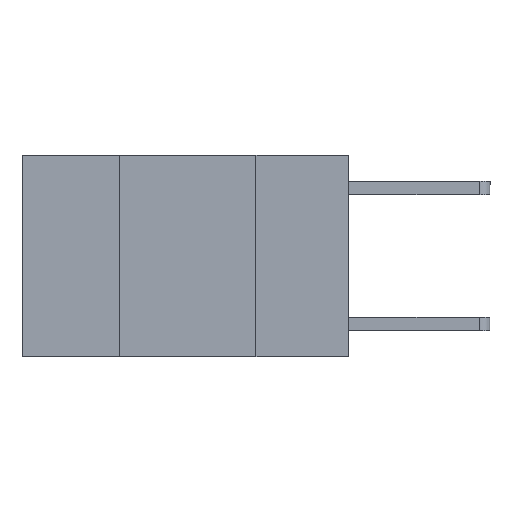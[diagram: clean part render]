
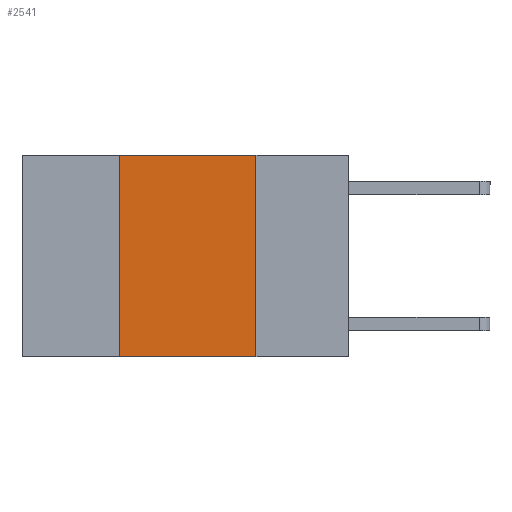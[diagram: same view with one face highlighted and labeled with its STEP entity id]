
A CAD part, left-side view. The second image highlights one B-rep face of the part: STEP entity #2541.
In plain terms, the highlighted planar face has unit normal (-1, 0, 0).
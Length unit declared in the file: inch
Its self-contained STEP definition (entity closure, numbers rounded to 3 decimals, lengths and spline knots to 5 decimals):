
#80 = EDGE_CURVE ( 'NONE', #4789, #7160, #1687, .T. ) ;
#711 = PLANE ( 'NONE',  #1277 ) ;
#1277 = AXIS2_PLACEMENT_3D ( 'NONE', #4644, #6618, #3279 ) ;
#1426 = FACE_OUTER_BOUND ( 'NONE', #3355, .T. ) ;
#1687 = LINE ( 'NONE', #3032, #4207 ) ;
#1963 = DIRECTION ( 'NONE',  ( 0., -1., 0. ) ) ;
#2150 = ORIENTED_EDGE ( 'NONE', *, *, #5941, .F. ) ;
#2434 = ORIENTED_EDGE ( 'NONE', *, *, #80, .F. ) ;
#2537 = LINE ( 'NONE', #5081, #6661 ) ;
#2541 = ADVANCED_FACE ( 'NONE', ( #1426 ), #711, .F. ) ;
#2850 = EDGE_CURVE ( 'NONE', #4996, #7160, #3863, .T. ) ;
#3003 = ORIENTED_EDGE ( 'NONE', *, *, #5790, .F. ) ;
#3032 = CARTESIAN_POINT ( 'NONE',  ( 0., 0.17, 0. ) ) ;
#3279 = DIRECTION ( 'NONE',  ( 0., 0., -1. ) ) ;
#3355 = EDGE_LOOP ( 'NONE', ( #2434, #2150, #3003, #3996 ) ) ;
#3646 = CARTESIAN_POINT ( 'NONE',  ( 0., 0.42, -0.37 ) ) ;
#3863 = LINE ( 'NONE', #7173, #7485 ) ;
#3996 = ORIENTED_EDGE ( 'NONE', *, *, #2850, .T. ) ;
#4000 = CARTESIAN_POINT ( 'NONE',  ( 0., 0.17, 0. ) ) ;
#4141 = VERTEX_POINT ( 'NONE', #6929 ) ;
#4207 = VECTOR ( 'NONE', #5582, 39.37008 ) ;
#4644 = CARTESIAN_POINT ( 'NONE',  ( 0., 0.6, 0. ) ) ;
#4751 = LINE ( 'NONE', #5539, #6401 ) ;
#4789 = VERTEX_POINT ( 'NONE', #4000 ) ;
#4996 = VERTEX_POINT ( 'NONE', #3646 ) ;
#5081 = CARTESIAN_POINT ( 'NONE',  ( 0., 0.6, 0. ) ) ;
#5539 = CARTESIAN_POINT ( 'NONE',  ( 0., 0.42, 0. ) ) ;
#5582 = DIRECTION ( 'NONE',  ( 0., 0., -1. ) ) ;
#5790 = EDGE_CURVE ( 'NONE', #4996, #4141, #4751, .T. ) ;
#5941 = EDGE_CURVE ( 'NONE', #4141, #4789, #2537, .T. ) ;
#6401 = VECTOR ( 'NONE', #6847, 39.37008 ) ;
#6618 = DIRECTION ( 'NONE',  ( 1., 0., 0. ) ) ;
#6661 = VECTOR ( 'NONE', #7607, 39.37008 ) ;
#6847 = DIRECTION ( 'NONE',  ( 0., 0., 1. ) ) ;
#6929 = CARTESIAN_POINT ( 'NONE',  ( 0., 0.42, 0. ) ) ;
#7160 = VERTEX_POINT ( 'NONE', #7624 ) ;
#7173 = CARTESIAN_POINT ( 'NONE',  ( 0., 0.6, -0.37 ) ) ;
#7485 = VECTOR ( 'NONE', #1963, 39.37008 ) ;
#7607 = DIRECTION ( 'NONE',  ( 0., -1., 0. ) ) ;
#7624 = CARTESIAN_POINT ( 'NONE',  ( 0., 0.17, -0.37 ) ) ;
